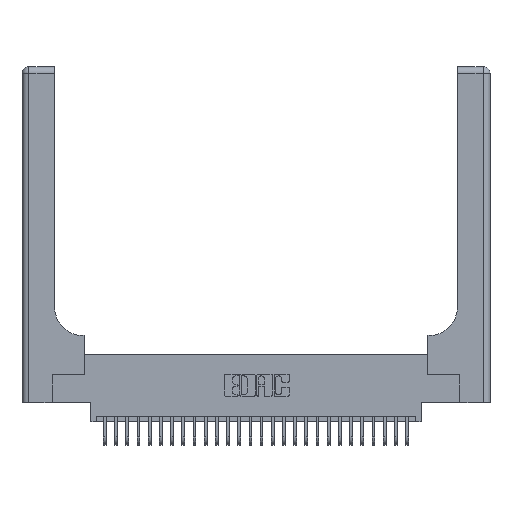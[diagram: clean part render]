
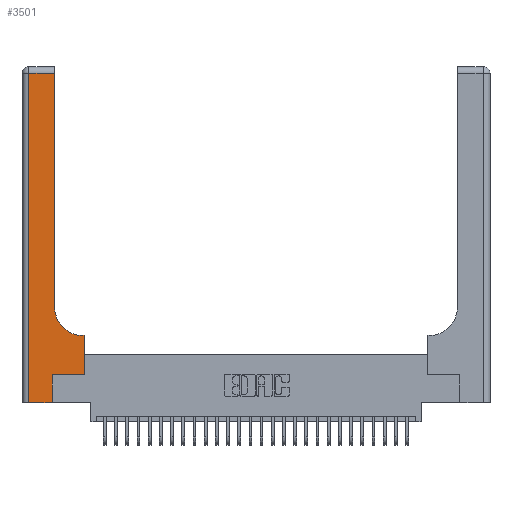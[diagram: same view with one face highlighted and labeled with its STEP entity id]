
A CAD part, top view. The second image highlights one B-rep face of the part: STEP entity #3501.
In plain terms, the highlighted planar face has unit normal (0, 0, 1).
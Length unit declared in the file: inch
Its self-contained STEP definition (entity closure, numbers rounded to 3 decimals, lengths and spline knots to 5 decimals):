
#649 = VECTOR ( 'NONE', #21461, 39.37008 ) ;
#787 = EDGE_CURVE ( 'NONE', #17407, #10871, #13572, .T. ) ;
#1079 = VERTEX_POINT ( 'NONE', #3929 ) ;
#1350 = DIRECTION ( 'NONE',  ( 1., 0., 0. ) ) ;
#1463 = LINE ( 'NONE', #7759, #7149 ) ;
#1701 = LINE ( 'NONE', #23660, #13726 ) ;
#2050 = CARTESIAN_POINT ( 'NONE',  ( 0.5415, 0.85, 0.37 ) ) ;
#2136 = LINE ( 'NONE', #25212, #26722 ) ;
#2230 = ORIENTED_EDGE ( 'NONE', *, *, #787, .T. ) ;
#2456 = VERTEX_POINT ( 'NONE', #10264 ) ;
#3501 = ADVANCED_FACE ( 'NONE', ( #26710 ), #6641, .F. ) ;
#3545 = EDGE_LOOP ( 'NONE', ( #25102, #25003, #2230, #19409, #8889, #20320, #19559, #12193, #6659 ) ) ;
#3929 = CARTESIAN_POINT ( 'NONE',  ( 0.5585, 0.6, 0.37 ) ) ;
#4478 = DIRECTION ( 'NONE',  ( 1., 0., 0. ) ) ;
#4816 = CARTESIAN_POINT ( 'NONE',  ( 0.269, 0., 0.37 ) ) ;
#5048 = DIRECTION ( 'NONE',  ( 1., 0., 0. ) ) ;
#5155 = VECTOR ( 'NONE', #5048, 39.37008 ) ;
#6641 = PLANE ( 'NONE',  #27011 ) ;
#6659 = ORIENTED_EDGE ( 'NONE', *, *, #16458, .T. ) ;
#7088 = VECTOR ( 'NONE', #18996, 39.37008 ) ;
#7147 = CARTESIAN_POINT ( 'NONE',  ( 0.2915, 3., 0.37 ) ) ;
#7149 = VECTOR ( 'NONE', #26719, 39.37008 ) ;
#7223 = VECTOR ( 'NONE', #11439, 39.37008 ) ;
#7528 = DIRECTION ( 'NONE',  ( -1., 0., 0. ) ) ;
#7759 = CARTESIAN_POINT ( 'NONE',  ( 0.2915, 0.6, 0.37 ) ) ;
#8889 = ORIENTED_EDGE ( 'NONE', *, *, #9755, .T. ) ;
#9744 = EDGE_CURVE ( 'NONE', #2456, #11755, #13424, .T. ) ;
#9755 = EDGE_CURVE ( 'NONE', #17618, #10742, #19731, .T. ) ;
#9916 = CARTESIAN_POINT ( 'NONE',  ( 0.06, 3., 0.37 ) ) ;
#10177 = LINE ( 'NONE', #21732, #16470 ) ;
#10264 = CARTESIAN_POINT ( 'NONE',  ( 0.2915, 0.85, 0.37 ) ) ;
#10531 = EDGE_CURVE ( 'NONE', #10871, #17618, #17819, .T. ) ;
#10742 = VERTEX_POINT ( 'NONE', #29532 ) ;
#10745 = CARTESIAN_POINT ( 'NONE',  ( 0.06, 2.94, 0.37 ) ) ;
#10871 = VERTEX_POINT ( 'NONE', #22803 ) ;
#11432 = DIRECTION ( 'NONE',  ( -1., 0., 0. ) ) ;
#11439 = DIRECTION ( 'NONE',  ( 0., -1., 0. ) ) ;
#11755 = VERTEX_POINT ( 'NONE', #19262 ) ;
#11848 = DIRECTION ( 'NONE',  ( 0., 1., 0. ) ) ;
#12193 = ORIENTED_EDGE ( 'NONE', *, *, #14346, .T. ) ;
#12264 = CARTESIAN_POINT ( 'NONE',  ( 0., 0., 0.37 ) ) ;
#13047 = EDGE_CURVE ( 'NONE', #11755, #17407, #10177, .T. ) ;
#13348 = CARTESIAN_POINT ( 'NONE',  ( 0.5585, 0.25, 0.37 ) ) ;
#13424 = LINE ( 'NONE', #7147, #7088 ) ;
#13572 = LINE ( 'NONE', #9916, #7223 ) ;
#13726 = VECTOR ( 'NONE', #11848, 39.37008 ) ;
#13868 = CARTESIAN_POINT ( 'NONE',  ( 0.5415, 0.6, 0.37 ) ) ;
#14346 = EDGE_CURVE ( 'NONE', #1079, #21485, #1463, .T. ) ;
#15666 = EDGE_CURVE ( 'NONE', #10742, #27135, #2136, .T. ) ;
#16458 = EDGE_CURVE ( 'NONE', #21485, #2456, #30370, .T. ) ;
#16470 = VECTOR ( 'NONE', #7528, 39.37008 ) ;
#16817 = AXIS2_PLACEMENT_3D ( 'NONE', #2050, #18778, #4478 ) ;
#17407 = VERTEX_POINT ( 'NONE', #10745 ) ;
#17618 = VERTEX_POINT ( 'NONE', #30386 ) ;
#17819 = LINE ( 'NONE', #12264, #5155 ) ;
#18778 = DIRECTION ( 'NONE',  ( 0., 0., -1. ) ) ;
#18996 = DIRECTION ( 'NONE',  ( 0., 1., 0. ) ) ;
#19262 = CARTESIAN_POINT ( 'NONE',  ( 0.2915, 2.94, 0.37 ) ) ;
#19409 = ORIENTED_EDGE ( 'NONE', *, *, #10531, .T. ) ;
#19559 = ORIENTED_EDGE ( 'NONE', *, *, #26140, .T. ) ;
#19731 = LINE ( 'NONE', #4816, #649 ) ;
#20320 = ORIENTED_EDGE ( 'NONE', *, *, #15666, .T. ) ;
#21461 = DIRECTION ( 'NONE',  ( 0., 1., 0. ) ) ;
#21485 = VERTEX_POINT ( 'NONE', #13868 ) ;
#21732 = CARTESIAN_POINT ( 'NONE',  ( 0., 2.94, 0.37 ) ) ;
#22803 = CARTESIAN_POINT ( 'NONE',  ( 0.06, 0., 0.37 ) ) ;
#23244 = CARTESIAN_POINT ( 'NONE',  ( 0., 3., 0.37 ) ) ;
#23660 = CARTESIAN_POINT ( 'NONE',  ( 0.5585, 0.25, 0.37 ) ) ;
#25003 = ORIENTED_EDGE ( 'NONE', *, *, #13047, .T. ) ;
#25102 = ORIENTED_EDGE ( 'NONE', *, *, #9744, .T. ) ;
#25212 = CARTESIAN_POINT ( 'NONE',  ( 0.269, 0.25, 0.37 ) ) ;
#25604 = DIRECTION ( 'NONE',  ( 0., 0., -1. ) ) ;
#26140 = EDGE_CURVE ( 'NONE', #27135, #1079, #1701, .T. ) ;
#26710 = FACE_OUTER_BOUND ( 'NONE', #3545, .T. ) ;
#26719 = DIRECTION ( 'NONE',  ( -1., 0., 0. ) ) ;
#26722 = VECTOR ( 'NONE', #1350, 39.37008 ) ;
#27011 = AXIS2_PLACEMENT_3D ( 'NONE', #23244, #25604, #11432 ) ;
#27135 = VERTEX_POINT ( 'NONE', #13348 ) ;
#29532 = CARTESIAN_POINT ( 'NONE',  ( 0.269, 0.25, 0.37 ) ) ;
#30370 = CIRCLE ( 'NONE', #16817, 0.25 ) ;
#30386 = CARTESIAN_POINT ( 'NONE',  ( 0.269, 0., 0.37 ) ) ;
